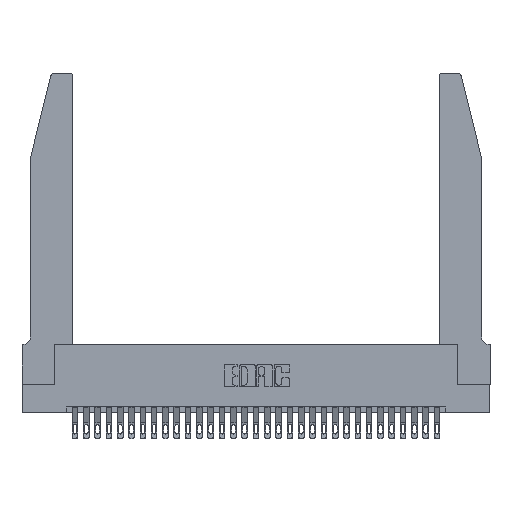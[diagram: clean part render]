
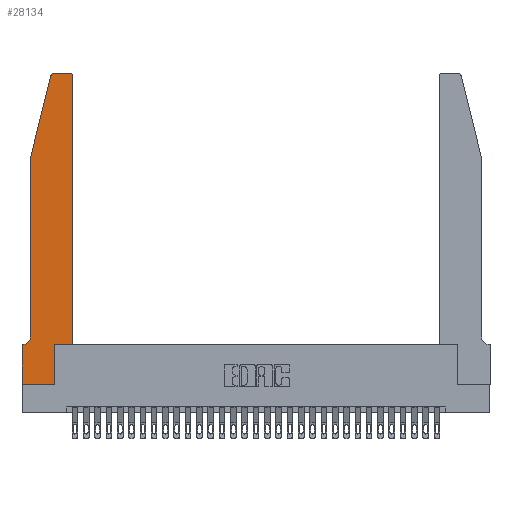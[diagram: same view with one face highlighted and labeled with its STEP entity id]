
A CAD part, top view. The second image highlights one B-rep face of the part: STEP entity #28134.
In plain terms, the highlighted planar face has unit normal (0, 0, 1).
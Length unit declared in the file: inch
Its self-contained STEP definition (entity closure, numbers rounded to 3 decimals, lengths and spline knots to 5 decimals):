
#344 = CARTESIAN_POINT ( 'NONE',  ( 0.2865, 0.35, 0.37 ) ) ;
#677 = CARTESIAN_POINT ( 'NONE',  ( 0.0755, 0.42, 0.37 ) ) ;
#1238 = DIRECTION ( 'NONE',  ( -1., 0., 0. ) ) ;
#1463 = EDGE_CURVE ( 'NONE', #31351, #23000, #23839, .T. ) ;
#1789 = DIRECTION ( 'NONE',  ( 0., 0., 1. ) ) ;
#1865 = EDGE_CURVE ( 'NONE', #17532, #21402, #4802, .T. ) ;
#2060 = EDGE_CURVE ( 'NONE', #14006, #12982, #13490, .T. ) ;
#2109 = VERTEX_POINT ( 'NONE', #2786 ) ;
#2786 = CARTESIAN_POINT ( 'NONE',  ( 0.4205, 2.75, 0.37 ) ) ;
#3010 = DIRECTION ( 'NONE',  ( 0., 1., 0. ) ) ;
#3104 = CARTESIAN_POINT ( 'NONE',  ( 0.0755, 2., 0.37 ) ) ;
#3321 = VECTOR ( 'NONE', #5693, 39.37008 ) ;
#3583 = CARTESIAN_POINT ( 'NONE',  ( 0.4505, 0.35, 0.37 ) ) ;
#3729 = CARTESIAN_POINT ( 'NONE',  ( 0.4505, 2.72, 0.37 ) ) ;
#3806 = DIRECTION ( 'NONE',  ( -1., 0., 0. ) ) ;
#3821 = DIRECTION ( 'NONE',  ( 0., 1., 0. ) ) ;
#3926 = CARTESIAN_POINT ( 'NONE',  ( 0.284, 2.72, 0.37 ) ) ;
#4147 = DIRECTION ( 'NONE',  ( 0., 0., 1. ) ) ;
#4388 = DIRECTION ( 'NONE',  ( -1., 0., 0. ) ) ;
#4633 = EDGE_LOOP ( 'NONE', ( #20303, #23266, #28598, #7099, #13496, #30682, #25102, #11765, #5300, #21289, #28962, #7640 ) ) ;
#4802 = LINE ( 'NONE', #344, #30345 ) ;
#5006 = DIRECTION ( 'NONE',  ( 0., 0., 1. ) ) ;
#5198 = FACE_OUTER_BOUND ( 'NONE', #4633, .T. ) ;
#5236 = VERTEX_POINT ( 'NONE', #677 ) ;
#5300 = ORIENTED_EDGE ( 'NONE', *, *, #1865, .T. ) ;
#5693 = DIRECTION ( 'NONE',  ( 0., -1., 0. ) ) ;
#6520 = CARTESIAN_POINT ( 'NONE',  ( 0.4505, 0.35, 0.37 ) ) ;
#6667 = VECTOR ( 'NONE', #4388, 39.37008 ) ;
#7087 = LINE ( 'NONE', #31154, #24507 ) ;
#7099 = ORIENTED_EDGE ( 'NONE', *, *, #19527, .T. ) ;
#7640 = ORIENTED_EDGE ( 'NONE', *, *, #23698, .T. ) ;
#8220 = VERTEX_POINT ( 'NONE', #17760 ) ;
#8767 = EDGE_CURVE ( 'NONE', #21402, #31351, #25734, .T. ) ;
#8919 = DIRECTION ( 'NONE',  ( 1., 0., 0. ) ) ;
#9666 = LINE ( 'NONE', #28625, #29297 ) ;
#11437 = EDGE_CURVE ( 'NONE', #8220, #30388, #19903, .T. ) ;
#11765 = ORIENTED_EDGE ( 'NONE', *, *, #30224, .T. ) ;
#11819 = CARTESIAN_POINT ( 'NONE',  ( 0.2865, 0.35, 0.37 ) ) ;
#12385 = VERTEX_POINT ( 'NONE', #21974 ) ;
#12542 = CARTESIAN_POINT ( 'NONE',  ( 0., 0., 0.37 ) ) ;
#12738 = VECTOR ( 'NONE', #23862, 39.37008 ) ;
#12982 = VERTEX_POINT ( 'NONE', #28808 ) ;
#13490 = CIRCLE ( 'NONE', #31277, 0.03 ) ;
#13496 = ORIENTED_EDGE ( 'NONE', *, *, #30831, .T. ) ;
#14006 = VERTEX_POINT ( 'NONE', #20473 ) ;
#14024 = DIRECTION ( 'NONE',  ( 1., 0., 0. ) ) ;
#14503 = CARTESIAN_POINT ( 'NONE',  ( 0.2865, 0., 0.37 ) ) ;
#15096 = VECTOR ( 'NONE', #26425, 39.37008 ) ;
#15216 = EDGE_CURVE ( 'NONE', #12982, #12385, #15408, .T. ) ;
#15408 = LINE ( 'NONE', #19968, #27644 ) ;
#16339 = DIRECTION ( 'NONE',  ( 0., 0., -1. ) ) ;
#16570 = VECTOR ( 'NONE', #3010, 39.37008 ) ;
#16704 = LINE ( 'NONE', #3104, #3321 ) ;
#16864 = CARTESIAN_POINT ( 'NONE',  ( 0.4205, 2.72, 0.37 ) ) ;
#17532 = VERTEX_POINT ( 'NONE', #14503 ) ;
#17760 = CARTESIAN_POINT ( 'NONE',  ( 0.0055, 0.35, 0.37 ) ) ;
#18172 = AXIS2_PLACEMENT_3D ( 'NONE', #31018, #16339, #1238 ) ;
#19070 = CARTESIAN_POINT ( 'NONE',  ( 0., 0., 0.37 ) ) ;
#19114 = CARTESIAN_POINT ( 'NONE',  ( 0., 0.35, 0.37 ) ) ;
#19332 = DIRECTION ( 'NONE',  ( 1., 0., 0. ) ) ;
#19527 = EDGE_CURVE ( 'NONE', #12385, #5236, #16704, .T. ) ;
#19903 = LINE ( 'NONE', #24254, #6667 ) ;
#19968 = CARTESIAN_POINT ( 'NONE',  ( 0.0755, 2., 0.37 ) ) ;
#20303 = ORIENTED_EDGE ( 'NONE', *, *, #21790, .T. ) ;
#20473 = CARTESIAN_POINT ( 'NONE',  ( 0.284, 2.75, 0.37 ) ) ;
#21289 = ORIENTED_EDGE ( 'NONE', *, *, #8767, .T. ) ;
#21402 = VERTEX_POINT ( 'NONE', #11819 ) ;
#21559 = DIRECTION ( 'NONE',  ( 1., 0., 0. ) ) ;
#21790 = EDGE_CURVE ( 'NONE', #2109, #14006, #9666, .T. ) ;
#21923 = CARTESIAN_POINT ( 'NONE',  ( 0., 0.35, 0.37 ) ) ;
#21974 = CARTESIAN_POINT ( 'NONE',  ( 0.0755, 2., 0.37 ) ) ;
#22316 = CIRCLE ( 'NONE', #23509, 0.03 ) ;
#22504 = EDGE_CURVE ( 'NONE', #30388, #29844, #23890, .T. ) ;
#23000 = VERTEX_POINT ( 'NONE', #3729 ) ;
#23266 = ORIENTED_EDGE ( 'NONE', *, *, #2060, .T. ) ;
#23509 = AXIS2_PLACEMENT_3D ( 'NONE', #16864, #1789, #19332 ) ;
#23698 = EDGE_CURVE ( 'NONE', #23000, #2109, #22316, .T. ) ;
#23787 = AXIS2_PLACEMENT_3D ( 'NONE', #19114, #4147, #21559 ) ;
#23811 = PLANE ( 'NONE',  #23787 ) ;
#23839 = LINE ( 'NONE', #3583, #16570 ) ;
#23862 = DIRECTION ( 'NONE',  ( 1., 0., 0. ) ) ;
#23890 = LINE ( 'NONE', #19070, #15096 ) ;
#24254 = CARTESIAN_POINT ( 'NONE',  ( 0.0755, 0.35, 0.37 ) ) ;
#24507 = VECTOR ( 'NONE', #14024, 39.37008 ) ;
#25102 = ORIENTED_EDGE ( 'NONE', *, *, #22504, .T. ) ;
#25734 = LINE ( 'NONE', #6520, #12738 ) ;
#26425 = DIRECTION ( 'NONE',  ( 0., -1., 0. ) ) ;
#27233 = DIRECTION ( 'NONE',  ( -0.239, -0.971, 0. ) ) ;
#27644 = VECTOR ( 'NONE', #27233, 39.37008 ) ;
#28134 = ADVANCED_FACE ( 'NONE', ( #5198 ), #23811, .T. ) ;
#28598 = ORIENTED_EDGE ( 'NONE', *, *, #15216, .T. ) ;
#28625 = CARTESIAN_POINT ( 'NONE',  ( 0.2605, 2.75, 0.37 ) ) ;
#28808 = CARTESIAN_POINT ( 'NONE',  ( 0.25487, 2.72718, 0.37 ) ) ;
#28962 = ORIENTED_EDGE ( 'NONE', *, *, #1463, .T. ) ;
#29297 = VECTOR ( 'NONE', #3806, 39.37008 ) ;
#29844 = VERTEX_POINT ( 'NONE', #12542 ) ;
#30224 = EDGE_CURVE ( 'NONE', #29844, #17532, #7087, .T. ) ;
#30345 = VECTOR ( 'NONE', #3821, 39.37008 ) ;
#30388 = VERTEX_POINT ( 'NONE', #21923 ) ;
#30435 = CARTESIAN_POINT ( 'NONE',  ( 0.4505, 0.35, 0.37 ) ) ;
#30682 = ORIENTED_EDGE ( 'NONE', *, *, #11437, .T. ) ;
#30831 = EDGE_CURVE ( 'NONE', #5236, #8220, #32142, .T. ) ;
#31018 = CARTESIAN_POINT ( 'NONE',  ( 0.0055, 0.42, 0.37 ) ) ;
#31154 = CARTESIAN_POINT ( 'NONE',  ( 0., 0., 0.37 ) ) ;
#31277 = AXIS2_PLACEMENT_3D ( 'NONE', #3926, #5006, #8919 ) ;
#31351 = VERTEX_POINT ( 'NONE', #30435 ) ;
#32142 = CIRCLE ( 'NONE', #18172, 0.07 ) ;
